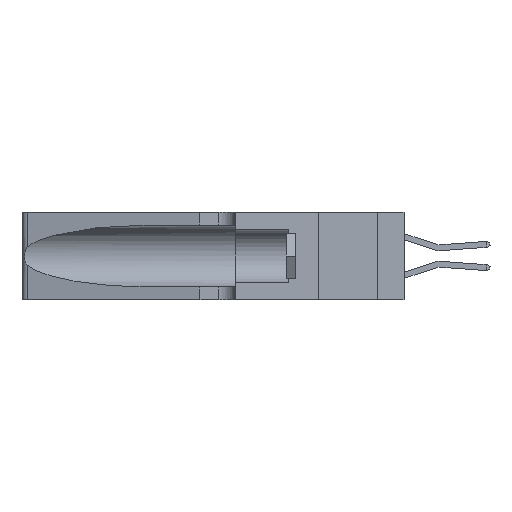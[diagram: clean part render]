
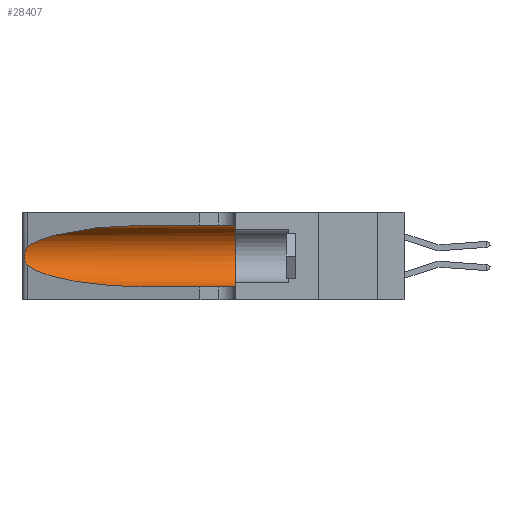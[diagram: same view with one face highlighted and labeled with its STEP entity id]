
A CAD part, left-side view. The second image highlights one B-rep face of the part: STEP entity #28407.
In plain terms, the highlighted cylindrical face has radius 3.308 mm (diameter 6.617 mm), a partial arc.
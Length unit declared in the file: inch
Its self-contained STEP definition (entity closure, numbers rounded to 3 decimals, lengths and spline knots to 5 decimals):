
#123 = CARTESIAN_POINT ( 'NONE',  ( 0.1305, 0.72297, 0.31525 ) ) ;
#552 = ORIENTED_EDGE ( 'NONE', *, *, #5110, .T. ) ;
#879 = DIRECTION ( 'NONE',  ( 0., -1., 0. ) ) ;
#1275 = ORIENTED_EDGE ( 'NONE', *, *, #6194, .F. ) ;
#1637 = FACE_OUTER_BOUND ( 'NONE', #18620, .T. ) ;
#1656 = CARTESIAN_POINT ( 'NONE',  ( 0.25639, 1.23184, 0.21858 ) ) ;
#1745 = CARTESIAN_POINT ( 'NONE',  ( 0.25789, 1.23486, 0.15765 ) ) ;
#1806 = LINE ( 'NONE', #27589, #13073 ) ;
#2372 = EDGE_CURVE ( 'NONE', #19142, #25162, #8001, .T. ) ;
#2418 = VERTEX_POINT ( 'NONE', #19743 ) ;
#2702 = CARTESIAN_POINT ( 'NONE',  ( 0.1305, 0.72297, 0.05475 ) ) ;
#2965 = DIRECTION ( 'NONE',  ( 0., -1., 0. ) ) ;
#2997 = CARTESIAN_POINT ( 'NONE',  ( 0.1305, 0.72297, 0.05475 ) ) ;
#3060 = CARTESIAN_POINT ( 'NONE',  ( 0.1305, 1.61858, 0.185 ) ) ;
#4055 = CARTESIAN_POINT ( 'NONE',  ( 0.25555, 1.22993, 0.14849 ) ) ;
#4331 = CARTESIAN_POINT ( 'NONE',  ( 0.2373, 1.15595, 0.28018 ) ) ;
#4711 = ORIENTED_EDGE ( 'NONE', *, *, #26300, .T. ) ;
#5110 = EDGE_CURVE ( 'NONE', #21654, #17286, #22417, .T. ) ;
#5257 = DIRECTION ( 'NONE',  ( 0., -1., 0. ) ) ;
#5739 = AXIS2_PLACEMENT_3D ( 'NONE', #19771, #6499, #21985 ) ;
#6168 = CARTESIAN_POINT ( 'NONE',  ( 0.25555, 1.22994, 0.2215 ) ) ;
#6194 = EDGE_CURVE ( 'NONE', #2418, #17286, #7828, .T. ) ;
#6499 = DIRECTION ( 'NONE',  ( 0., 1., 0. ) ) ;
#7828 = CIRCLE ( 'NONE', #5739, 0.13025 ) ;
#8001 = B_SPLINE_CURVE_WITH_KNOTS ( 'NONE', 3,
 ( #21764, #6168, #1656, #8515, #23989, #10748, #26201, #12983, #28424, #15193, #1745, #17454, #4055, #19649 ),
 .UNSPECIFIED., .F., .F.,
 ( 4, 2, 2, 2, 2, 2, 4 ),
 ( 0., 0.00027, 0.00053, 0.00107, 0.0016, 0.00187, 0.00214 ),
 .UNSPECIFIED. ) ;
#8515 = CARTESIAN_POINT ( 'NONE',  ( 0.25787, 1.23484, 0.2124 ) ) ;
#9722 = CARTESIAN_POINT ( 'NONE',  ( 0.2373, 1.15595, 0.08982 ) ) ;
#10748 = CARTESIAN_POINT ( 'NONE',  ( 0.26018, 1.23835, 0.19895 ) ) ;
#11019 =( BOUNDED_CURVE ( )  B_SPLINE_CURVE ( 3, ( #26469, #15462, #4331, #19907 ),
 .UNSPECIFIED., .F., .F. ) 
 B_SPLINE_CURVE_WITH_KNOTS ( ( 4, 4 ),
 ( 1.5708, 2.84003 ),
 .UNSPECIFIED. ) 
 CURVE ( )  GEOMETRIC_REPRESENTATION_ITEM ( )  RATIONAL_B_SPLINE_CURVE ( ( 1., 0.87, 0.87, 1. ) ) 
 REPRESENTATION_ITEM ( '' )  );
#11359 = VECTOR ( 'NONE', #5257, 39.37008 ) ;
#12275 = ORIENTED_EDGE ( 'NONE', *, *, #15213, .F. ) ;
#12983 = CARTESIAN_POINT ( 'NONE',  ( 0.26075, 1.23896, 0.178 ) ) ;
#13073 = VECTOR ( 'NONE', #879, 39.37008 ) ;
#14924 = CARTESIAN_POINT ( 'NONE',  ( 0.1305, 0.35, 0.05475 ) ) ;
#15193 = CARTESIAN_POINT ( 'NONE',  ( 0.25856, 1.23593, 0.16098 ) ) ;
#15213 = EDGE_CURVE ( 'NONE', #20334, #2418, #1806, .T. ) ;
#15462 = CARTESIAN_POINT ( 'NONE',  ( 0.18966, 0.96281, 0.31525 ) ) ;
#16216 = CARTESIAN_POINT ( 'NONE',  ( 0.25487, 1.22718, 0.22369 ) ) ;
#16235 = EDGE_CURVE ( 'NONE', #20334, #19142, #11019, .T. ) ;
#16325 = CARTESIAN_POINT ( 'NONE',  ( 0.25487, 1.22718, 0.14631 ) ) ;
#16425 = CARTESIAN_POINT ( 'NONE',  ( 0.18966, 0.96281, 0.05475 ) ) ;
#16888 = ORIENTED_EDGE ( 'NONE', *, *, #16235, .T. ) ;
#17286 = VERTEX_POINT ( 'NONE', #14924 ) ;
#17454 = CARTESIAN_POINT ( 'NONE',  ( 0.25639, 1.23186, 0.15144 ) ) ;
#18575 = CARTESIAN_POINT ( 'NONE',  ( 0.1305, 1.61858, 0.05475 ) ) ;
#18620 = EDGE_LOOP ( 'NONE', ( #16888, #27923, #4711, #552, #1275, #12275 ) ) ;
#18710 = DIRECTION ( 'NONE',  ( 0., 0., -1. ) ) ;
#18809 = CYLINDRICAL_SURFACE ( 'NONE', #22996, 0.13025 ) ;
#19142 = VERTEX_POINT ( 'NONE', #16216 ) ;
#19201 =( BOUNDED_CURVE ( )  B_SPLINE_CURVE ( 3, ( #16325, #9722, #16425, #2997 ),
 .UNSPECIFIED., .F., .F. ) 
 B_SPLINE_CURVE_WITH_KNOTS ( ( 4, 4 ),
 ( 3.44316, 4.71239 ),
 .UNSPECIFIED. ) 
 CURVE ( )  GEOMETRIC_REPRESENTATION_ITEM ( )  RATIONAL_B_SPLINE_CURVE ( ( 1., 0.87, 0.87, 1. ) ) 
 REPRESENTATION_ITEM ( '' )  );
#19649 = CARTESIAN_POINT ( 'NONE',  ( 0.25487, 1.22718, 0.14631 ) ) ;
#19743 = CARTESIAN_POINT ( 'NONE',  ( 0.1305, 0.35, 0.31525 ) ) ;
#19771 = CARTESIAN_POINT ( 'NONE',  ( 0.1305, 0.35, 0.185 ) ) ;
#19907 = CARTESIAN_POINT ( 'NONE',  ( 0.25487, 1.22718, 0.22369 ) ) ;
#20334 = VERTEX_POINT ( 'NONE', #123 ) ;
#21654 = VERTEX_POINT ( 'NONE', #2702 ) ;
#21764 = CARTESIAN_POINT ( 'NONE',  ( 0.25487, 1.22718, 0.22369 ) ) ;
#21985 = DIRECTION ( 'NONE',  ( 0., 0., 1. ) ) ;
#22417 = LINE ( 'NONE', #18575, #11359 ) ;
#22996 = AXIS2_PLACEMENT_3D ( 'NONE', #3060, #2965, #18710 ) ;
#23989 = CARTESIAN_POINT ( 'NONE',  ( 0.25854, 1.2359, 0.20912 ) ) ;
#25162 = VERTEX_POINT ( 'NONE', #27853 ) ;
#26201 = CARTESIAN_POINT ( 'NONE',  ( 0.26075, 1.23896, 0.19203 ) ) ;
#26300 = EDGE_CURVE ( 'NONE', #25162, #21654, #19201, .T. ) ;
#26469 = CARTESIAN_POINT ( 'NONE',  ( 0.1305, 0.72297, 0.31525 ) ) ;
#27589 = CARTESIAN_POINT ( 'NONE',  ( 0.1305, 1.61858, 0.31525 ) ) ;
#27853 = CARTESIAN_POINT ( 'NONE',  ( 0.25487, 1.22718, 0.14631 ) ) ;
#27923 = ORIENTED_EDGE ( 'NONE', *, *, #2372, .T. ) ;
#28407 = ADVANCED_FACE ( 'NONE', ( #1637 ), #18809, .F. ) ;
#28424 = CARTESIAN_POINT ( 'NONE',  ( 0.26017, 1.23833, 0.17102 ) ) ;
